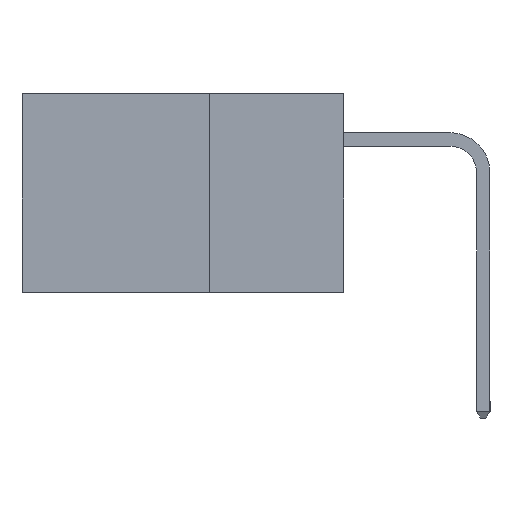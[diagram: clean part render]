
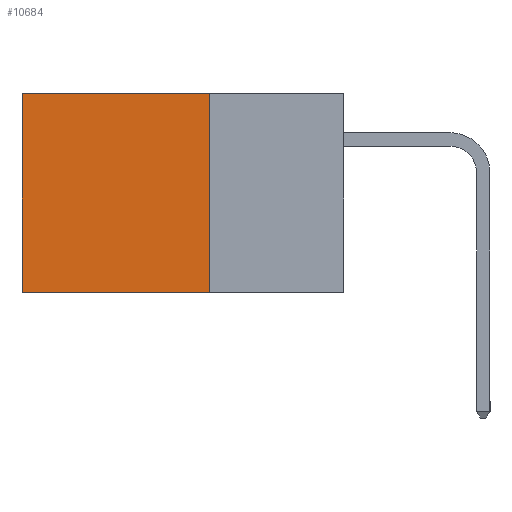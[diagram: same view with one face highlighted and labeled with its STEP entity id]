
A CAD part, left-side view. The second image highlights one B-rep face of the part: STEP entity #10684.
In plain terms, the highlighted planar face has unit normal (-1, 0, 0).
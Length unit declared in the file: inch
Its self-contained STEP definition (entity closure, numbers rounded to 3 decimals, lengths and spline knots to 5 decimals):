
#79 = ORIENTED_EDGE ( 'NONE', *, *, #872, .F. ) ;
#233 = CARTESIAN_POINT ( 'NONE',  ( 0.2615, 0.25, 0. ) ) ;
#325 = DIRECTION ( 'NONE',  ( 1., 0., 0. ) ) ;
#372 = PLANE ( 'NONE',  #9629 ) ;
#542 = CARTESIAN_POINT ( 'NONE',  ( 0.2615, 0.25, -0.37 ) ) ;
#872 = EDGE_CURVE ( 'NONE', #7976, #7584, #11039, .T. ) ;
#1232 = VECTOR ( 'NONE', #7546, 39.37008 ) ;
#1481 = CARTESIAN_POINT ( 'NONE',  ( 0.2615, 0.25, -0.37 ) ) ;
#1702 = ORIENTED_EDGE ( 'NONE', *, *, #4785, .T. ) ;
#2371 = CARTESIAN_POINT ( 'NONE',  ( 0.2615, 0.25, -0.37 ) ) ;
#2378 = DIRECTION ( 'NONE',  ( 0., 1., 0. ) ) ;
#3016 = VERTEX_POINT ( 'NONE', #8371 ) ;
#3056 = CARTESIAN_POINT ( 'NONE',  ( 0.2615, 0.25, 0. ) ) ;
#4015 = LINE ( 'NONE', #4883, #8465 ) ;
#4785 = EDGE_CURVE ( 'NONE', #3016, #7584, #4015, .T. ) ;
#4883 = CARTESIAN_POINT ( 'NONE',  ( 0.2615, 0.6, -0.37 ) ) ;
#4965 = LINE ( 'NONE', #233, #9106 ) ;
#5038 = CARTESIAN_POINT ( 'NONE',  ( 0.2615, 0.6, -0.37 ) ) ;
#5912 = VECTOR ( 'NONE', #8005, 39.37008 ) ;
#5971 = EDGE_CURVE ( 'NONE', #7530, #3016, #4965, .T. ) ;
#6741 = EDGE_LOOP ( 'NONE', ( #1702, #79, #11291, #7688 ) ) ;
#6966 = DIRECTION ( 'NONE',  ( 0., 0., -1. ) ) ;
#7530 = VERTEX_POINT ( 'NONE', #3056 ) ;
#7546 = DIRECTION ( 'NONE',  ( 0., 0., -1. ) ) ;
#7584 = VERTEX_POINT ( 'NONE', #5038 ) ;
#7688 = ORIENTED_EDGE ( 'NONE', *, *, #5971, .T. ) ;
#7976 = VERTEX_POINT ( 'NONE', #11312 ) ;
#8005 = DIRECTION ( 'NONE',  ( 0., 1., 0. ) ) ;
#8371 = CARTESIAN_POINT ( 'NONE',  ( 0.2615, 0.6, 0. ) ) ;
#8465 = VECTOR ( 'NONE', #6966, 39.37008 ) ;
#8956 = EDGE_CURVE ( 'NONE', #7530, #7976, #12498, .T. ) ;
#9106 = VECTOR ( 'NONE', #2378, 39.37008 ) ;
#9629 = AXIS2_PLACEMENT_3D ( 'NONE', #1481, #325, #13053 ) ;
#10684 = ADVANCED_FACE ( 'NONE', ( #12093 ), #372, .F. ) ;
#11039 = LINE ( 'NONE', #542, #5912 ) ;
#11291 = ORIENTED_EDGE ( 'NONE', *, *, #8956, .F. ) ;
#11312 = CARTESIAN_POINT ( 'NONE',  ( 0.2615, 0.25, -0.37 ) ) ;
#12093 = FACE_OUTER_BOUND ( 'NONE', #6741, .T. ) ;
#12498 = LINE ( 'NONE', #2371, #1232 ) ;
#13053 = DIRECTION ( 'NONE',  ( 0., 0., -1. ) ) ;
